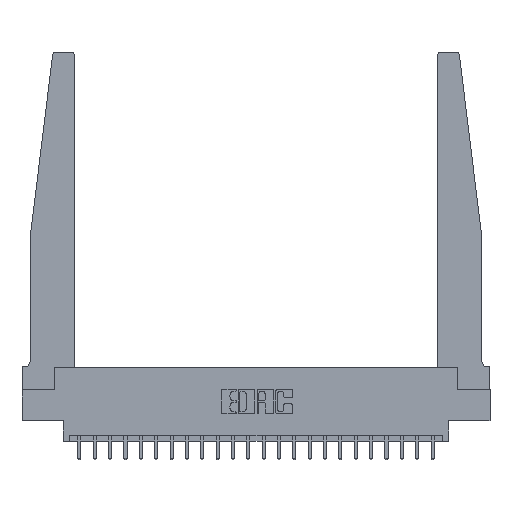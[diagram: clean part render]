
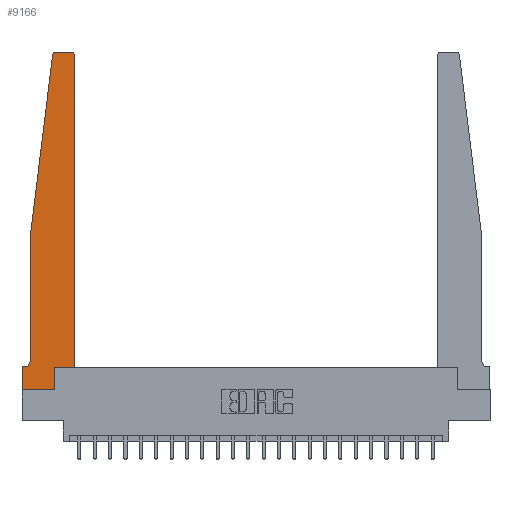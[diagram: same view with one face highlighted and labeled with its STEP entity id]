
A CAD part, top view. The second image highlights one B-rep face of the part: STEP entity #9166.
In plain terms, the highlighted planar face has unit normal (0, 0, 1).
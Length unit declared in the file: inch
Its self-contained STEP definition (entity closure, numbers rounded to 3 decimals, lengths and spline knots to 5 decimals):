
#42 = EDGE_CURVE ( 'NONE', #16303, #13292, #3177, .T. ) ;
#59 = EDGE_CURVE ( 'NONE', #9374, #17559, #10002, .T. ) ;
#94 = DIRECTION ( 'NONE',  ( 0., 0., 1. ) ) ;
#343 = CARTESIAN_POINT ( 'NONE',  ( 0.425, 0.18, 0.37 ) ) ;
#510 = CIRCLE ( 'NONE', #16779, 0.03 ) ;
#531 = DIRECTION ( 'NONE',  ( 0., 0., -1. ) ) ;
#542 = CARTESIAN_POINT ( 'NONE',  ( 0.2605, 0.18, 0.37 ) ) ;
#745 = CARTESIAN_POINT ( 'NONE',  ( 0.065, 1.25, 0.37 ) ) ;
#797 = CARTESIAN_POINT ( 'NONE',  ( 0., 0., 0.37 ) ) ;
#913 = DIRECTION ( 'NONE',  ( 1., 0., 0. ) ) ;
#1138 = EDGE_CURVE ( 'NONE', #9663, #7292, #16742, .T. ) ;
#1300 = VERTEX_POINT ( 'NONE', #13295 ) ;
#1523 = ORIENTED_EDGE ( 'NONE', *, *, #20621, .T. ) ;
#2236 = CARTESIAN_POINT ( 'NONE',  ( 0.395, 2.72, 0.37 ) ) ;
#2350 = DIRECTION ( 'NONE',  ( 1., 0., 0. ) ) ;
#2614 = EDGE_CURVE ( 'NONE', #1300, #9663, #22570, .T. ) ;
#2690 = LINE ( 'NONE', #16913, #3715 ) ;
#3043 = EDGE_CURVE ( 'NONE', #10207, #9374, #13273, .T. ) ;
#3177 = LINE ( 'NONE', #6404, #16817 ) ;
#3211 = LINE ( 'NONE', #10452, #22342 ) ;
#3365 = VECTOR ( 'NONE', #3955, 39.37008 ) ;
#3715 = VECTOR ( 'NONE', #22377, 39.37008 ) ;
#3955 = DIRECTION ( 'NONE',  ( -0.122, -0.992, 0. ) ) ;
#4308 = CARTESIAN_POINT ( 'NONE',  ( 0.425, 0.18, 0.37 ) ) ;
#4616 = ORIENTED_EDGE ( 'NONE', *, *, #22939, .T. ) ;
#4618 = CARTESIAN_POINT ( 'NONE',  ( 0.25, 2.75, 0.37 ) ) ;
#4645 = CARTESIAN_POINT ( 'NONE',  ( 0.065, 0.1875, 0.37 ) ) ;
#4887 = CARTESIAN_POINT ( 'NONE',  ( 0.2605, 0., 0.37 ) ) ;
#5437 = EDGE_CURVE ( 'NONE', #7165, #10207, #510, .T. ) ;
#5446 = ORIENTED_EDGE ( 'NONE', *, *, #19371, .T. ) ;
#5831 = DIRECTION ( 'NONE',  ( 0., -1., 0. ) ) ;
#5854 = CARTESIAN_POINT ( 'NONE',  ( 0., 0., 0.37 ) ) ;
#6404 = CARTESIAN_POINT ( 'NONE',  ( 0.2605, 0.18, 0.37 ) ) ;
#6703 = DIRECTION ( 'NONE',  ( 0., 0., 1. ) ) ;
#7165 = VERTEX_POINT ( 'NONE', #15729 ) ;
#7292 = VERTEX_POINT ( 'NONE', #5854 ) ;
#7786 = DIRECTION ( 'NONE',  ( -1., 0., 0. ) ) ;
#7844 = CARTESIAN_POINT ( 'NONE',  ( 0., 0.1875, 0.37 ) ) ;
#8483 = PLANE ( 'NONE',  #17253 ) ;
#8528 = DIRECTION ( 'NONE',  ( 0., 0., 1. ) ) ;
#8606 = FACE_OUTER_BOUND ( 'NONE', #14754, .T. ) ;
#8945 = ORIENTED_EDGE ( 'NONE', *, *, #59, .T. ) ;
#9166 = ADVANCED_FACE ( 'NONE', ( #8606 ), #8483, .T. ) ;
#9374 = VERTEX_POINT ( 'NONE', #10346 ) ;
#9475 = DIRECTION ( 'NONE',  ( 1., 0., 0. ) ) ;
#9663 = VERTEX_POINT ( 'NONE', #7844 ) ;
#10002 = CIRCLE ( 'NONE', #23264, 0.03 ) ;
#10006 = EDGE_CURVE ( 'NONE', #17654, #1300, #10478, .T. ) ;
#10207 = VERTEX_POINT ( 'NONE', #14282 ) ;
#10346 = CARTESIAN_POINT ( 'NONE',  ( 0.27653, 2.75, 0.37 ) ) ;
#10452 = CARTESIAN_POINT ( 'NONE',  ( 0.065, 1.25, 0.37 ) ) ;
#10478 = CIRCLE ( 'NONE', #15388, 0.05 ) ;
#10550 = ORIENTED_EDGE ( 'NONE', *, *, #20042, .T. ) ;
#10710 = VECTOR ( 'NONE', #20900, 39.37008 ) ;
#11379 = ORIENTED_EDGE ( 'NONE', *, *, #42, .T. ) ;
#11971 = DIRECTION ( 'NONE',  ( 0., 1., 0. ) ) ;
#12093 = CARTESIAN_POINT ( 'NONE',  ( 0.27653, 2.72, 0.37 ) ) ;
#12244 = ORIENTED_EDGE ( 'NONE', *, *, #13827, .T. ) ;
#13273 = LINE ( 'NONE', #4618, #15254 ) ;
#13292 = VERTEX_POINT ( 'NONE', #542 ) ;
#13295 = CARTESIAN_POINT ( 'NONE',  ( 0.015, 0.1875, 0.37 ) ) ;
#13554 = ORIENTED_EDGE ( 'NONE', *, *, #2614, .T. ) ;
#13827 = EDGE_CURVE ( 'NONE', #18793, #17654, #3211, .T. ) ;
#14015 = CARTESIAN_POINT ( 'NONE',  ( 0.065, 0.2375, 0.37 ) ) ;
#14282 = CARTESIAN_POINT ( 'NONE',  ( 0.395, 2.75, 0.37 ) ) ;
#14754 = EDGE_LOOP ( 'NONE', ( #21567, #8945, #1523, #12244, #21209, #13554, #21277, #4616, #11379, #5446, #10550, #23290 ) ) ;
#14858 = CARTESIAN_POINT ( 'NONE',  ( 0.065, 1.25, 0.37 ) ) ;
#14978 = LINE ( 'NONE', #14858, #3365 ) ;
#15254 = VECTOR ( 'NONE', #17071, 39.37008 ) ;
#15388 = AXIS2_PLACEMENT_3D ( 'NONE', #16781, #531, #7786 ) ;
#15401 = LINE ( 'NONE', #797, #19487 ) ;
#15729 = CARTESIAN_POINT ( 'NONE',  ( 0.425, 2.72, 0.37 ) ) ;
#16203 = VECTOR ( 'NONE', #2350, 39.37008 ) ;
#16303 = VERTEX_POINT ( 'NONE', #4887 ) ;
#16742 = LINE ( 'NONE', #22091, #20811 ) ;
#16779 = AXIS2_PLACEMENT_3D ( 'NONE', #2236, #94, #9475 ) ;
#16781 = CARTESIAN_POINT ( 'NONE',  ( 0.015, 0.2375, 0.37 ) ) ;
#16817 = VECTOR ( 'NONE', #11971, 39.37008 ) ;
#16913 = CARTESIAN_POINT ( 'NONE',  ( 0.425, 0.18, 0.37 ) ) ;
#17071 = DIRECTION ( 'NONE',  ( -1., 0., 0. ) ) ;
#17253 = AXIS2_PLACEMENT_3D ( 'NONE', #17597, #6703, #21640 ) ;
#17414 = VERTEX_POINT ( 'NONE', #4308 ) ;
#17559 = VERTEX_POINT ( 'NONE', #22812 ) ;
#17597 = CARTESIAN_POINT ( 'NONE',  ( 0., 0.1875, 0.37 ) ) ;
#17654 = VERTEX_POINT ( 'NONE', #14015 ) ;
#17676 = DIRECTION ( 'NONE',  ( 0., -1., 0. ) ) ;
#18793 = VERTEX_POINT ( 'NONE', #745 ) ;
#19371 = EDGE_CURVE ( 'NONE', #13292, #17414, #22162, .T. ) ;
#19487 = VECTOR ( 'NONE', #913, 39.37008 ) ;
#20042 = EDGE_CURVE ( 'NONE', #17414, #7165, #2690, .T. ) ;
#20621 = EDGE_CURVE ( 'NONE', #17559, #18793, #14978, .T. ) ;
#20811 = VECTOR ( 'NONE', #5831, 39.37008 ) ;
#20863 = DIRECTION ( 'NONE',  ( 1., 0., 0. ) ) ;
#20900 = DIRECTION ( 'NONE',  ( -1., 0., 0. ) ) ;
#21209 = ORIENTED_EDGE ( 'NONE', *, *, #10006, .T. ) ;
#21277 = ORIENTED_EDGE ( 'NONE', *, *, #1138, .T. ) ;
#21567 = ORIENTED_EDGE ( 'NONE', *, *, #3043, .T. ) ;
#21640 = DIRECTION ( 'NONE',  ( 1., 0., 0. ) ) ;
#22091 = CARTESIAN_POINT ( 'NONE',  ( 0., 0., 0.37 ) ) ;
#22162 = LINE ( 'NONE', #343, #16203 ) ;
#22342 = VECTOR ( 'NONE', #17676, 39.37008 ) ;
#22377 = DIRECTION ( 'NONE',  ( 0., 1., 0. ) ) ;
#22570 = LINE ( 'NONE', #4645, #10710 ) ;
#22812 = CARTESIAN_POINT ( 'NONE',  ( 0.24675, 2.72367, 0.37 ) ) ;
#22939 = EDGE_CURVE ( 'NONE', #7292, #16303, #15401, .T. ) ;
#23264 = AXIS2_PLACEMENT_3D ( 'NONE', #12093, #8528, #20863 ) ;
#23290 = ORIENTED_EDGE ( 'NONE', *, *, #5437, .T. ) ;
